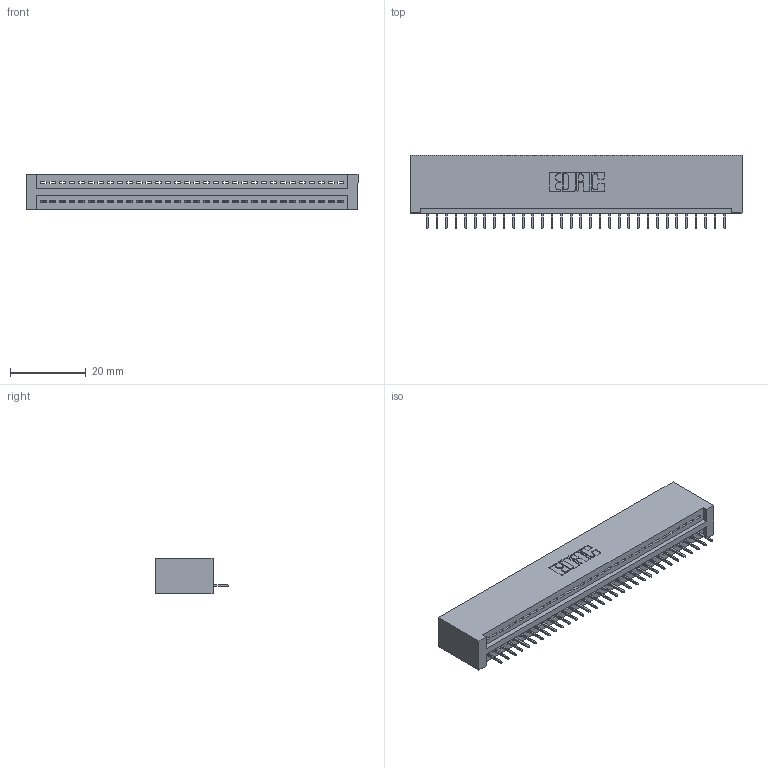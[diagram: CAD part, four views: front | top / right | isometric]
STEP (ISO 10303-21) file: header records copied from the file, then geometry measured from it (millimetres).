
FILE_DESCRIPTION (( 'STEP AP203' ), '1' );
FILE_NAME ('395-032-524-101.STEP', '2018-11-12T19:16:46', ( '' ), ( '' ), 'SwSTEP 2.0', 'SolidWorks 2016', '' );
FILE_SCHEMA (( 'CONFIG_CONTROL_DESIGN' ));
Length unit declared in the file: inch
Products named in the file (3): 345-292-001_345-293-124; 345 Part_No Mounting Lugs; 395-032-524-101
Assembly tree (33 placements, depth 2):
  395-032-524-101
    345 Part_No Mounting Lugs
    345-292-001_345-293-124  x32
Bounding box: 87.88 x 19.35 x 9.4 mm (x, y, z)
Volume: 8723.3 mm3; surface area: 11242.6 mm2
Topology: 33 solids, 33 shells, 2102 faces, 6077 edges, 3922 vertices
Faces by surface type: plane 1548, cylinder 554
Entity records: 25227 total; most frequent: CARTESIAN_POINT 4376, ORIENTED_EDGE 4342, DIRECTION 3831, EDGE_CURVE 2171, VECTOR 1923, LINE 1923, VERTEX_POINT 1442, AXIS2_PLACEMENT_3D 954
